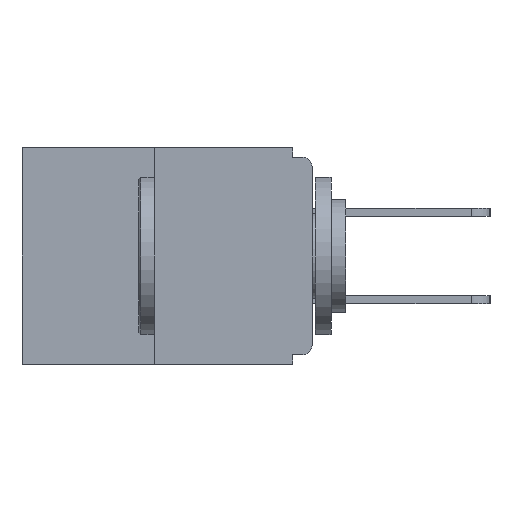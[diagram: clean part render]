
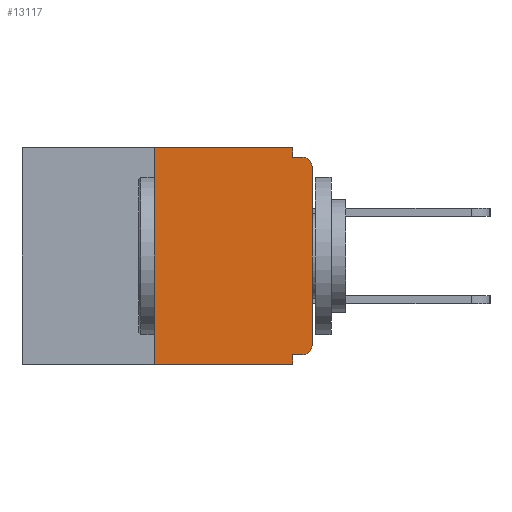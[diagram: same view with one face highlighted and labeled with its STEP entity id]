
A CAD part, left-side view. The second image highlights one B-rep face of the part: STEP entity #13117.
In plain terms, the highlighted planar face has unit normal (-1, 0, 0).
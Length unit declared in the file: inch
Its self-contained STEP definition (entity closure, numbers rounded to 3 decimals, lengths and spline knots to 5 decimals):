
#604 = VECTOR ( 'NONE', #17859, 39.37008 ) ;
#739 = ORIENTED_EDGE ( 'NONE', *, *, #2205, .T. ) ;
#933 = VECTOR ( 'NONE', #15339, 39.37008 ) ;
#1035 = CARTESIAN_POINT ( 'NONE',  ( 0., 0.015, -0.03 ) ) ;
#1167 = AXIS2_PLACEMENT_3D ( 'NONE', #12933, #6881, #9873 ) ;
#1358 = DIRECTION ( 'NONE',  ( 0., 0., -1. ) ) ;
#1724 = FACE_OUTER_BOUND ( 'NONE', #13365, .T. ) ;
#2205 = EDGE_CURVE ( 'NONE', #7322, #17810, #16817, .T. ) ;
#2353 = VECTOR ( 'NONE', #1358, 39.37008 ) ;
#2562 = DIRECTION ( 'NONE',  ( 0., 0., -1. ) ) ;
#2620 = CARTESIAN_POINT ( 'NONE',  ( 0., 0., -0.03 ) ) ;
#3012 = VECTOR ( 'NONE', #15544, 39.37008 ) ;
#3212 = DIRECTION ( 'NONE',  ( 0., 0., 1. ) ) ;
#3386 = VECTOR ( 'NONE', #10650, 39.37008 ) ;
#3397 = EDGE_CURVE ( 'NONE', #7322, #9437, #8010, .T. ) ;
#3703 = PLANE ( 'NONE',  #16837 ) ;
#3846 = ORIENTED_EDGE ( 'NONE', *, *, #13741, .F. ) ;
#3916 = ORIENTED_EDGE ( 'NONE', *, *, #17861, .F. ) ;
#4353 = CARTESIAN_POINT ( 'NONE',  ( 0., 0.46, 0. ) ) ;
#4939 = ORIENTED_EDGE ( 'NONE', *, *, #5758, .T. ) ;
#5608 = AXIS2_PLACEMENT_3D ( 'NONE', #1035, #7339, #2562 ) ;
#5758 = EDGE_CURVE ( 'NONE', #18401, #8091, #16718, .T. ) ;
#5781 = VECTOR ( 'NONE', #17471, 39.37008 ) ;
#5794 = CARTESIAN_POINT ( 'NONE',  ( 0., 0.031, -0.015 ) ) ;
#6881 = DIRECTION ( 'NONE',  ( -1., 0., 0. ) ) ;
#6897 = LINE ( 'NONE', #8895, #2353 ) ;
#6918 = VERTEX_POINT ( 'NONE', #16892 ) ;
#7006 = CARTESIAN_POINT ( 'NONE',  ( 0., 0.015, -0.328 ) ) ;
#7055 = LINE ( 'NONE', #15475, #3012 ) ;
#7160 = VERTEX_POINT ( 'NONE', #11935 ) ;
#7185 = EDGE_CURVE ( 'NONE', #10943, #16442, #12336, .T. ) ;
#7322 = VERTEX_POINT ( 'NONE', #7899 ) ;
#7339 = DIRECTION ( 'NONE',  ( -1., 0., 0. ) ) ;
#7459 = CARTESIAN_POINT ( 'NONE',  ( 0., 0.031, -0.328 ) ) ;
#7899 = CARTESIAN_POINT ( 'NONE',  ( 0., 0.25, -0.343 ) ) ;
#8010 = LINE ( 'NONE', #18245, #14128 ) ;
#8091 = VERTEX_POINT ( 'NONE', #19362 ) ;
#8187 = VERTEX_POINT ( 'NONE', #5794 ) ;
#8557 = EDGE_CURVE ( 'NONE', #10943, #6918, #8799, .T. ) ;
#8799 = CIRCLE ( 'NONE', #1167, 0.015 ) ;
#8807 = DIRECTION ( 'NONE',  ( 1., 0., 0. ) ) ;
#8895 = CARTESIAN_POINT ( 'NONE',  ( 0., 0.031, 0. ) ) ;
#9103 = CARTESIAN_POINT ( 'NONE',  ( 0., 0., -0.328 ) ) ;
#9437 = VERTEX_POINT ( 'NONE', #11604 ) ;
#9873 = DIRECTION ( 'NONE',  ( 0., 0., -1. ) ) ;
#10474 = EDGE_CURVE ( 'NONE', #7160, #8187, #6897, .T. ) ;
#10650 = DIRECTION ( 'NONE',  ( 0., 0., 1. ) ) ;
#10722 = CARTESIAN_POINT ( 'NONE',  ( 0., 0.46, -0.343 ) ) ;
#10943 = VERTEX_POINT ( 'NONE', #7006 ) ;
#11220 = ORIENTED_EDGE ( 'NONE', *, *, #7185, .F. ) ;
#11604 = CARTESIAN_POINT ( 'NONE',  ( 0., 0.25, 0. ) ) ;
#11607 = LINE ( 'NONE', #16595, #3386 ) ;
#11758 = ORIENTED_EDGE ( 'NONE', *, *, #18198, .F. ) ;
#11868 = ORIENTED_EDGE ( 'NONE', *, *, #3397, .F. ) ;
#11935 = CARTESIAN_POINT ( 'NONE',  ( 0., 0.031, 0. ) ) ;
#12336 = LINE ( 'NONE', #9103, #18820 ) ;
#12591 = CARTESIAN_POINT ( 'NONE',  ( 0., 0., -0.015 ) ) ;
#12933 = CARTESIAN_POINT ( 'NONE',  ( 0., 0.015, -0.313 ) ) ;
#13117 = ADVANCED_FACE ( 'NONE', ( #1724 ), #3703, .F. ) ;
#13365 = EDGE_LOOP ( 'NONE', ( #11758, #11868, #739, #3916, #11220, #13859, #16000, #4939, #3846, #16792 ) ) ;
#13741 = EDGE_CURVE ( 'NONE', #8187, #8091, #14279, .T. ) ;
#13859 = ORIENTED_EDGE ( 'NONE', *, *, #8557, .T. ) ;
#14128 = VECTOR ( 'NONE', #3212, 39.37008 ) ;
#14279 = LINE ( 'NONE', #12591, #5781 ) ;
#14318 = EDGE_CURVE ( 'NONE', #6918, #18401, #11607, .T. ) ;
#15339 = DIRECTION ( 'NONE',  ( 0., -1., 0. ) ) ;
#15475 = CARTESIAN_POINT ( 'NONE',  ( 0., 0.031, -0.343 ) ) ;
#15544 = DIRECTION ( 'NONE',  ( 0., 0., -1. ) ) ;
#16000 = ORIENTED_EDGE ( 'NONE', *, *, #14318, .T. ) ;
#16442 = VERTEX_POINT ( 'NONE', #7459 ) ;
#16595 = CARTESIAN_POINT ( 'NONE',  ( 0., 0., 0. ) ) ;
#16718 = CIRCLE ( 'NONE', #5608, 0.015 ) ;
#16792 = ORIENTED_EDGE ( 'NONE', *, *, #10474, .F. ) ;
#16817 = LINE ( 'NONE', #10722, #933 ) ;
#16837 = AXIS2_PLACEMENT_3D ( 'NONE', #17720, #8807, #17904 ) ;
#16892 = CARTESIAN_POINT ( 'NONE',  ( 0., 0., -0.313 ) ) ;
#17463 = LINE ( 'NONE', #4353, #604 ) ;
#17471 = DIRECTION ( 'NONE',  ( 0., -1., 0. ) ) ;
#17720 = CARTESIAN_POINT ( 'NONE',  ( 0., 0.46, 0. ) ) ;
#17810 = VERTEX_POINT ( 'NONE', #18136 ) ;
#17859 = DIRECTION ( 'NONE',  ( 0., -1., 0. ) ) ;
#17861 = EDGE_CURVE ( 'NONE', #16442, #17810, #7055, .T. ) ;
#17904 = DIRECTION ( 'NONE',  ( 0., 0., -1. ) ) ;
#18023 = DIRECTION ( 'NONE',  ( 0., 1., 0. ) ) ;
#18136 = CARTESIAN_POINT ( 'NONE',  ( 0., 0.031, -0.343 ) ) ;
#18198 = EDGE_CURVE ( 'NONE', #9437, #7160, #17463, .T. ) ;
#18245 = CARTESIAN_POINT ( 'NONE',  ( 0., 0.25, 0. ) ) ;
#18401 = VERTEX_POINT ( 'NONE', #2620 ) ;
#18820 = VECTOR ( 'NONE', #18023, 39.37008 ) ;
#19362 = CARTESIAN_POINT ( 'NONE',  ( 0., 0.015, -0.015 ) ) ;
